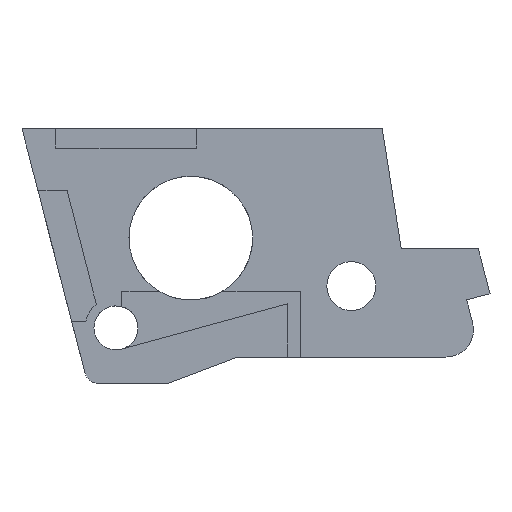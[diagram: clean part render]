
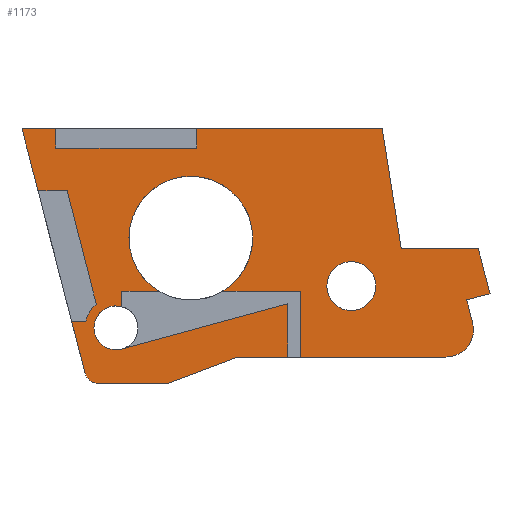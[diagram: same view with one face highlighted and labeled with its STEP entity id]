
A CAD part, left-side view. The second image highlights one B-rep face of the part: STEP entity #1173.
In plain terms, the highlighted planar face has unit normal (-1, 0, 0).
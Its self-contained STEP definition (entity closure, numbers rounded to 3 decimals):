
#26=FACE_BOUND('',#125,.T.);
#36=CIRCLE('',#1246,2.25);
#37=CIRCLE('',#1247,1.);
#38=CIRCLE('',#1248,1.6);
#39=CIRCLE('',#1249,4.5);
#40=CIRCLE('',#1250,4.5);
#41=CIRCLE('',#1251,2.);
#42=CIRCLE('',#1252,1.775);
#66=FACE_OUTER_BOUND('',#124,.T.);
#124=EDGE_LOOP('',(#790,#791,#792,#793,#794,#795,#796,#797,#798,#799,#800,
#801,#802,#803,#804,#805,#806,#807,#808,#809,#810,#811,#812,#813,#814,#815,
#816,#817,#818,#819,#820));
#125=EDGE_LOOP('',(#821));
#195=LINE('',#1662,#343);
#199=LINE('',#1670,#347);
#202=LINE('',#1676,#350);
#203=LINE('',#1678,#351);
#204=LINE('',#1680,#352);
#205=LINE('',#1682,#353);
#206=LINE('',#1684,#354);
#207=LINE('',#1686,#355);
#208=LINE('',#1688,#356);
#209=LINE('',#1690,#357);
#210=LINE('',#1694,#358);
#211=LINE('',#1696,#359);
#212=LINE('',#1700,#360);
#213=LINE('',#1702,#361);
#214=LINE('',#1704,#362);
#215=LINE('',#1706,#363);
#216=LINE('',#1708,#364);
#217=LINE('',#1712,#365);
#218=LINE('',#1714,#366);
#219=LINE('',#1720,#367);
#220=LINE('',#1722,#368);
#221=LINE('',#1724,#369);
#222=LINE('',#1728,#370);
#223=LINE('',#1730,#371);
#224=LINE('',#1731,#372);
#343=VECTOR('',#1340,10.);
#347=VECTOR('',#1346,10.);
#350=VECTOR('',#1351,10.);
#351=VECTOR('',#1352,10.);
#352=VECTOR('',#1353,10.);
#353=VECTOR('',#1354,10.);
#354=VECTOR('',#1355,10.);
#355=VECTOR('',#1356,10.);
#356=VECTOR('',#1357,10.);
#357=VECTOR('',#1358,10.);
#358=VECTOR('',#1361,10.);
#359=VECTOR('',#1362,10.);
#360=VECTOR('',#1365,10.);
#361=VECTOR('',#1366,10.);
#362=VECTOR('',#1367,10.);
#363=VECTOR('',#1368,10.);
#364=VECTOR('',#1369,10.);
#365=VECTOR('',#1372,10.);
#366=VECTOR('',#1373,10.);
#367=VECTOR('',#1378,10.);
#368=VECTOR('',#1379,10.);
#369=VECTOR('',#1380,10.);
#370=VECTOR('',#1383,10.);
#371=VECTOR('',#1384,10.);
#372=VECTOR('',#1385,10.);
#490=VERTEX_POINT('',#1660);
#491=VERTEX_POINT('',#1661);
#494=VERTEX_POINT('',#1669);
#496=VERTEX_POINT('',#1675);
#497=VERTEX_POINT('',#1677);
#498=VERTEX_POINT('',#1679);
#499=VERTEX_POINT('',#1681);
#500=VERTEX_POINT('',#1683);
#501=VERTEX_POINT('',#1685);
#502=VERTEX_POINT('',#1687);
#503=VERTEX_POINT('',#1689);
#504=VERTEX_POINT('',#1691);
#505=VERTEX_POINT('',#1693);
#506=VERTEX_POINT('',#1695);
#507=VERTEX_POINT('',#1697);
#508=VERTEX_POINT('',#1699);
#509=VERTEX_POINT('',#1701);
#510=VERTEX_POINT('',#1703);
#511=VERTEX_POINT('',#1705);
#512=VERTEX_POINT('',#1707);
#513=VERTEX_POINT('',#1709);
#514=VERTEX_POINT('',#1711);
#515=VERTEX_POINT('',#1713);
#516=VERTEX_POINT('',#1715);
#517=VERTEX_POINT('',#1717);
#518=VERTEX_POINT('',#1719);
#519=VERTEX_POINT('',#1721);
#520=VERTEX_POINT('',#1723);
#521=VERTEX_POINT('',#1725);
#522=VERTEX_POINT('',#1727);
#523=VERTEX_POINT('',#1729);
#524=VERTEX_POINT('',#1732);
#607=EDGE_CURVE('',#490,#491,#195,.T.);
#611=EDGE_CURVE('',#494,#490,#199,.T.);
#614=EDGE_CURVE('',#491,#496,#202,.T.);
#615=EDGE_CURVE('',#496,#497,#203,.T.);
#616=EDGE_CURVE('',#497,#498,#204,.T.);
#617=EDGE_CURVE('',#498,#499,#205,.T.);
#618=EDGE_CURVE('',#499,#500,#206,.T.);
#619=EDGE_CURVE('',#500,#501,#207,.T.);
#620=EDGE_CURVE('',#501,#502,#208,.T.);
#621=EDGE_CURVE('',#502,#503,#209,.T.);
#622=EDGE_CURVE('',#503,#504,#36,.T.);
#623=EDGE_CURVE('',#504,#505,#210,.T.);
#624=EDGE_CURVE('',#505,#506,#211,.T.);
#625=EDGE_CURVE('',#507,#506,#37,.T.);
#626=EDGE_CURVE('',#507,#508,#212,.T.);
#627=EDGE_CURVE('',#509,#508,#213,.T.);
#628=EDGE_CURVE('',#510,#509,#214,.T.);
#629=EDGE_CURVE('',#510,#511,#215,.T.);
#630=EDGE_CURVE('',#511,#512,#216,.T.);
#631=EDGE_CURVE('',#513,#512,#38,.T.);
#632=EDGE_CURVE('',#513,#514,#217,.T.);
#633=EDGE_CURVE('',#514,#515,#218,.T.);
#634=EDGE_CURVE('',#516,#515,#39,.T.);
#635=EDGE_CURVE('',#517,#516,#40,.T.);
#636=EDGE_CURVE('',#517,#518,#219,.T.);
#637=EDGE_CURVE('',#518,#519,#220,.T.);
#638=EDGE_CURVE('',#520,#519,#221,.T.);
#639=EDGE_CURVE('',#521,#520,#41,.T.);
#640=EDGE_CURVE('',#521,#522,#222,.T.);
#641=EDGE_CURVE('',#523,#522,#223,.T.);
#642=EDGE_CURVE('',#494,#523,#224,.T.);
#643=EDGE_CURVE('',#524,#524,#42,.T.);
#790=ORIENTED_EDGE('',*,*,#611,.T.);
#791=ORIENTED_EDGE('',*,*,#607,.T.);
#792=ORIENTED_EDGE('',*,*,#614,.T.);
#793=ORIENTED_EDGE('',*,*,#615,.T.);
#794=ORIENTED_EDGE('',*,*,#616,.T.);
#795=ORIENTED_EDGE('',*,*,#617,.T.);
#796=ORIENTED_EDGE('',*,*,#618,.T.);
#797=ORIENTED_EDGE('',*,*,#619,.T.);
#798=ORIENTED_EDGE('',*,*,#620,.T.);
#799=ORIENTED_EDGE('',*,*,#621,.T.);
#800=ORIENTED_EDGE('',*,*,#622,.T.);
#801=ORIENTED_EDGE('',*,*,#623,.T.);
#802=ORIENTED_EDGE('',*,*,#624,.T.);
#803=ORIENTED_EDGE('',*,*,#625,.F.);
#804=ORIENTED_EDGE('',*,*,#626,.T.);
#805=ORIENTED_EDGE('',*,*,#627,.F.);
#806=ORIENTED_EDGE('',*,*,#628,.F.);
#807=ORIENTED_EDGE('',*,*,#629,.T.);
#808=ORIENTED_EDGE('',*,*,#630,.T.);
#809=ORIENTED_EDGE('',*,*,#631,.F.);
#810=ORIENTED_EDGE('',*,*,#632,.T.);
#811=ORIENTED_EDGE('',*,*,#633,.T.);
#812=ORIENTED_EDGE('',*,*,#634,.F.);
#813=ORIENTED_EDGE('',*,*,#635,.F.);
#814=ORIENTED_EDGE('',*,*,#636,.T.);
#815=ORIENTED_EDGE('',*,*,#637,.T.);
#816=ORIENTED_EDGE('',*,*,#638,.F.);
#817=ORIENTED_EDGE('',*,*,#639,.F.);
#818=ORIENTED_EDGE('',*,*,#640,.T.);
#819=ORIENTED_EDGE('',*,*,#641,.F.);
#820=ORIENTED_EDGE('',*,*,#642,.F.);
#821=ORIENTED_EDGE('',*,*,#643,.F.);
#1126=PLANE('',#1245);
#1173=ADVANCED_FACE('',(#66,#26),#1126,.F.);
#1245=AXIS2_PLACEMENT_3D('',#1674,#1349,#1350);
#1246=AXIS2_PLACEMENT_3D('',#1692,#1359,#1360);
#1247=AXIS2_PLACEMENT_3D('',#1698,#1363,#1364);
#1248=AXIS2_PLACEMENT_3D('',#1710,#1370,#1371);
#1249=AXIS2_PLACEMENT_3D('',#1716,#1374,#1375);
#1250=AXIS2_PLACEMENT_3D('',#1718,#1376,#1377);
#1251=AXIS2_PLACEMENT_3D('',#1726,#1381,#1382);
#1252=AXIS2_PLACEMENT_3D('',#1733,#1386,#1387);
#1340=DIRECTION('',(0.,0.157,0.988));
#1346=DIRECTION('',(0.,1.,0.));
#1349=DIRECTION('center_axis',(1.,0.,0.));
#1350=DIRECTION('ref_axis',(0.,1.,0.));
#1351=DIRECTION('',(0.,1.,0.));
#1352=DIRECTION('',(0.,0.,-1.));
#1353=DIRECTION('',(0.,1.,0.));
#1354=DIRECTION('',(0.,0.,1.));
#1355=DIRECTION('',(0.,1.,0.));
#1356=DIRECTION('',(0.,-0.25,-0.968));
#1357=DIRECTION('',(0.,-1.,0.));
#1358=DIRECTION('',(0.,-0.25,-0.968));
#1359=DIRECTION('center_axis',(-1.,0.,0.));
#1360=DIRECTION('ref_axis',(0.,1.,0.));
#1361=DIRECTION('',(0.,1.,0.));
#1362=DIRECTION('',(0.,-0.25,-0.968));
#1363=DIRECTION('center_axis',(1.,0.,0.));
#1364=DIRECTION('ref_axis',(0.,0.612,-0.79));
#1365=DIRECTION('',(0.,-1.,0.));
#1366=DIRECTION('',(0.,0.935,-0.354));
#1367=DIRECTION('',(0.,1.,0.));
#1368=DIRECTION('',(0.,0.,1.));
#1369=DIRECTION('',(0.,0.965,-0.264));
#1370=DIRECTION('center_axis',(-1.,0.,0.));
#1371=DIRECTION('ref_axis',(0.,1.,0.));
#1372=DIRECTION('',(0.,0.,1.));
#1373=DIRECTION('',(0.,-1.,0.));
#1374=DIRECTION('center_axis',(-1.,0.,0.));
#1375=DIRECTION('ref_axis',(0.,1.,0.));
#1376=DIRECTION('center_axis',(-1.,0.,0.));
#1377=DIRECTION('ref_axis',(0.,1.,0.));
#1378=DIRECTION('',(0.,-1.,0.));
#1379=DIRECTION('',(0.,0.,-1.));
#1380=DIRECTION('',(0.,1.,0.));
#1381=DIRECTION('center_axis',(1.,0.,0.));
#1382=DIRECTION('ref_axis',(0.,-0.79,-0.612));
#1383=DIRECTION('',(0.,0.25,0.968));
#1384=DIRECTION('',(0.,0.968,-0.25));
#1385=DIRECTION('',(0.,-0.25,-0.968));
#1386=DIRECTION('center_axis',(-1.,0.,0.));
#1387=DIRECTION('ref_axis',(0.,1.,0.));
#1660=CARTESIAN_POINT('',(0.,-0.134,2.707));
#1661=CARTESIAN_POINT('',(0.,1.251,11.437));
#1662=CARTESIAN_POINT('',(0.,0.648,7.635));
#1669=CARTESIAN_POINT('',(0.,-5.743,2.707));
#1670=CARTESIAN_POINT('',(0.,-8.672,2.707));
#1674=CARTESIAN_POINT('Origin',(0.,10.427,2.187));
#1675=CARTESIAN_POINT('',(0.,14.74,11.437));
#1676=CARTESIAN_POINT('',(0.,-3.491,11.437));
#1677=CARTESIAN_POINT('',(0.,14.74,10.037));
#1678=CARTESIAN_POINT('',(0.,14.74,6.112));
#1679=CARTESIAN_POINT('',(0.,24.99,10.037));
#1680=CARTESIAN_POINT('',(0.,17.708,10.037));
#1681=CARTESIAN_POINT('',(0.,24.99,11.437));
#1682=CARTESIAN_POINT('',(0.,24.99,6.812));
#1683=CARTESIAN_POINT('',(0.,27.44,11.437));
#1684=CARTESIAN_POINT('',(0.,-3.491,11.437));
#1685=CARTESIAN_POINT('',(0.,26.279,6.937));
#1686=CARTESIAN_POINT('',(0.,27.44,11.437));
#1687=CARTESIAN_POINT('',(0.,24.162,6.937));
#1688=CARTESIAN_POINT('',(0.,17.294,6.937));
#1689=CARTESIAN_POINT('',(0.,22.036,-1.305));
#1690=CARTESIAN_POINT('',(0.,22.096,-1.072));
#1691=CARTESIAN_POINT('',(0.,22.805,-2.563));
#1692=CARTESIAN_POINT('Origin',(0.,20.606,-3.043));
#1693=CARTESIAN_POINT('',(0.,23.828,-2.563));
#1694=CARTESIAN_POINT('',(0.,17.128,-2.563));
#1695=CARTESIAN_POINT('',(0.,22.861,-6.313));
#1696=CARTESIAN_POINT('',(0.,27.44,11.437));
#1697=CARTESIAN_POINT('',(0.,21.893,-7.063));
#1698=CARTESIAN_POINT('Origin',(0.,21.893,-6.063));
#1699=CARTESIAN_POINT('',(0.,16.78,-7.063));
#1700=CARTESIAN_POINT('',(0.,22.668,-7.063));
#1701=CARTESIAN_POINT('',(0.,11.757,-5.163));
#1702=CARTESIAN_POINT('',(0.,11.757,-5.163));
#1703=CARTESIAN_POINT('',(0.,8.106,-5.163));
#1704=CARTESIAN_POINT('',(0.,-7.773,-5.163));
#1705=CARTESIAN_POINT('',(0.,8.106,-1.283));
#1706=CARTESIAN_POINT('',(0.,8.106,-1.488));
#1707=CARTESIAN_POINT('',(0.,20.184,-4.586));
#1708=CARTESIAN_POINT('',(0.,8.744,-1.458));
#1709=CARTESIAN_POINT('',(0.,20.184,-1.5));
#1710=CARTESIAN_POINT('Origin',(0.,20.606,-3.043));
#1711=CARTESIAN_POINT('',(0.,20.184,-0.363));
#1712=CARTESIAN_POINT('',(0.,20.184,0.344));
#1713=CARTESIAN_POINT('',(0.,17.495,-0.363));
#1714=CARTESIAN_POINT('',(0.,15.306,-0.363));
#1715=CARTESIAN_POINT('',(0.,10.665,3.487));
#1716=CARTESIAN_POINT('Origin',(0.,15.165,3.487));
#1717=CARTESIAN_POINT('',(0.,12.835,-0.363));
#1718=CARTESIAN_POINT('Origin',(0.,15.165,3.487));
#1719=CARTESIAN_POINT('',(0.,7.186,-0.363));
#1720=CARTESIAN_POINT('',(0.,11.631,-0.363));
#1721=CARTESIAN_POINT('',(0.,7.186,-5.163));
#1722=CARTESIAN_POINT('',(0.,7.186,0.912));
#1723=CARTESIAN_POINT('',(0.,-3.384,-5.163));
#1724=CARTESIAN_POINT('',(0.,-7.773,-5.163));
#1725=CARTESIAN_POINT('',(0.,-5.321,-2.664));
#1726=CARTESIAN_POINT('Origin',(0.,-3.384,-3.163));
#1727=CARTESIAN_POINT('',(0.,-4.892,-1.));
#1728=CARTESIAN_POINT('',(0.,-6.455,-7.063));
#1729=CARTESIAN_POINT('',(0.,-6.586,-0.563));
#1730=CARTESIAN_POINT('',(0.,-6.586,-0.563));
#1731=CARTESIAN_POINT('',(0.,-3.491,11.437));
#1732=CARTESIAN_POINT('',(0.,1.725,0.));
#1733=CARTESIAN_POINT('Origin',(0.,3.5,0.));
